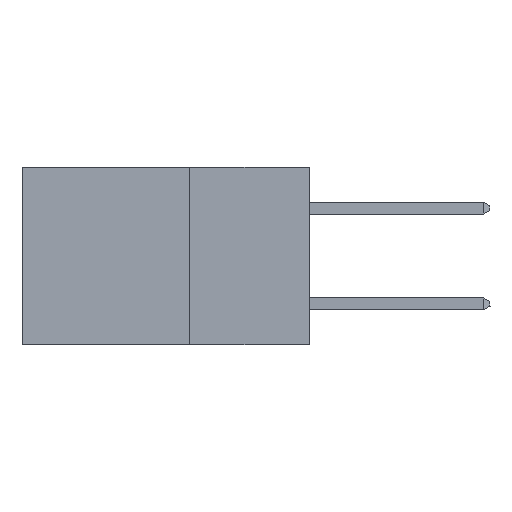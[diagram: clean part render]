
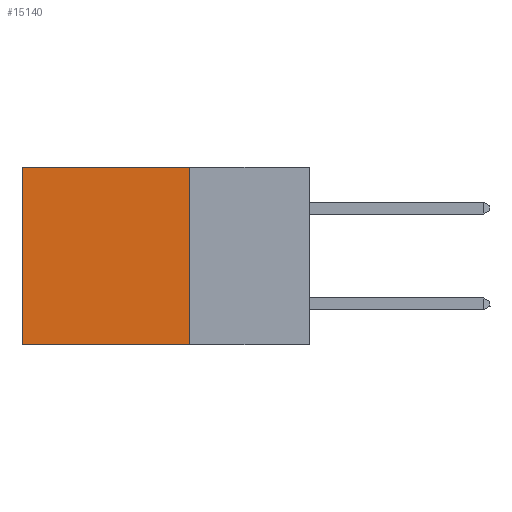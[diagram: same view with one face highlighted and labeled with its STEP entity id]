
A CAD part, left-side view. The second image highlights one B-rep face of the part: STEP entity #15140.
In plain terms, the highlighted planar face has unit normal (-1, 0, 0).
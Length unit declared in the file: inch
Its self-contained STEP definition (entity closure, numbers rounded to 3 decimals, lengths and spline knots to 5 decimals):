
#142 = DIRECTION ( 'NONE',  ( 0., 1., 0. ) ) ;
#346 = VECTOR ( 'NONE', #1695, 39.37008 ) ;
#1486 = LINE ( 'NONE', #7563, #17582 ) ;
#1531 = ORIENTED_EDGE ( 'NONE', *, *, #19877, .F. ) ;
#1695 = DIRECTION ( 'NONE',  ( 0., 0., -1. ) ) ;
#2427 = VERTEX_POINT ( 'NONE', #6633 ) ;
#3330 = ORIENTED_EDGE ( 'NONE', *, *, #4755, .F. ) ;
#3418 = DIRECTION ( 'NONE',  ( 0., 0., -1. ) ) ;
#4143 = EDGE_LOOP ( 'NONE', ( #11726, #1531, #3330, #22407 ) ) ;
#4755 = EDGE_CURVE ( 'NONE', #13523, #21986, #21634, .T. ) ;
#6633 = CARTESIAN_POINT ( 'NONE',  ( 0.2875, 0.6, -0.37 ) ) ;
#7000 = CARTESIAN_POINT ( 'NONE',  ( 0.2875, 0.6, 0. ) ) ;
#7155 = LINE ( 'NONE', #7000, #15334 ) ;
#7563 = CARTESIAN_POINT ( 'NONE',  ( 0.2875, 0.25, -0.37 ) ) ;
#7571 = DIRECTION ( 'NONE',  ( 1., 0., 0. ) ) ;
#7826 = CARTESIAN_POINT ( 'NONE',  ( 0.2875, 0.25, 0. ) ) ;
#10682 = LINE ( 'NONE', #12502, #19383 ) ;
#11726 = ORIENTED_EDGE ( 'NONE', *, *, #16769, .T. ) ;
#12502 = CARTESIAN_POINT ( 'NONE',  ( 0.2875, 0.25, 0. ) ) ;
#12815 = DIRECTION ( 'NONE',  ( 0., 0., -1. ) ) ;
#13523 = VERTEX_POINT ( 'NONE', #7826 ) ;
#13806 = CARTESIAN_POINT ( 'NONE',  ( 0.2875, 0.25, -0.37 ) ) ;
#14274 = VERTEX_POINT ( 'NONE', #15722 ) ;
#15140 = ADVANCED_FACE ( 'NONE', ( #20306 ), #19826, .F. ) ;
#15334 = VECTOR ( 'NONE', #3418, 39.37008 ) ;
#15722 = CARTESIAN_POINT ( 'NONE',  ( 0.2875, 0.6, 0. ) ) ;
#16396 = CARTESIAN_POINT ( 'NONE',  ( 0.2875, 0.25, 0. ) ) ;
#16769 = EDGE_CURVE ( 'NONE', #14274, #2427, #7155, .T. ) ;
#17108 = EDGE_CURVE ( 'NONE', #13523, #14274, #10682, .T. ) ;
#17467 = CARTESIAN_POINT ( 'NONE',  ( 0.2875, 0.25, 0. ) ) ;
#17582 = VECTOR ( 'NONE', #19743, 39.37008 ) ;
#18378 = AXIS2_PLACEMENT_3D ( 'NONE', #16396, #7571, #12815 ) ;
#19383 = VECTOR ( 'NONE', #142, 39.37008 ) ;
#19743 = DIRECTION ( 'NONE',  ( 0., 1., 0. ) ) ;
#19826 = PLANE ( 'NONE',  #18378 ) ;
#19877 = EDGE_CURVE ( 'NONE', #21986, #2427, #1486, .T. ) ;
#20306 = FACE_OUTER_BOUND ( 'NONE', #4143, .T. ) ;
#21634 = LINE ( 'NONE', #17467, #346 ) ;
#21986 = VERTEX_POINT ( 'NONE', #13806 ) ;
#22407 = ORIENTED_EDGE ( 'NONE', *, *, #17108, .T. ) ;
